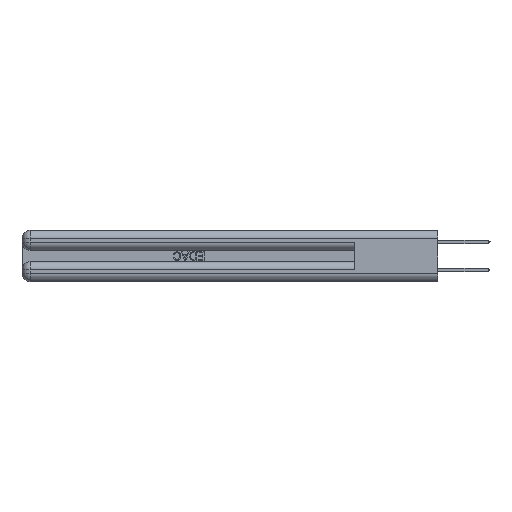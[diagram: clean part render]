
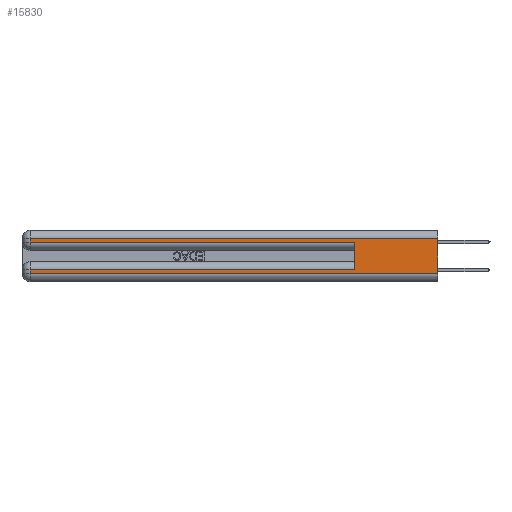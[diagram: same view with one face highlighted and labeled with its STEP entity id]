
A CAD part, left-side view. The second image highlights one B-rep face of the part: STEP entity #15830.
In plain terms, the highlighted planar face has unit normal (-1, 0, 0).
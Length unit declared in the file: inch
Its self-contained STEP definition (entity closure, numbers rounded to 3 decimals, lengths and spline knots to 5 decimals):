
#198 = DIRECTION ( 'NONE',  ( 1., 0., 0. ) ) ;
#2492 = DIRECTION ( 'NONE',  ( 0., 0., -1. ) ) ;
#3030 = CARTESIAN_POINT ( 'NONE',  ( 0., 2.94, 0.31 ) ) ;
#3040 = LINE ( 'NONE', #41547, #27461 ) ;
#3312 = EDGE_CURVE ( 'NONE', #23851, #37595, #28689, .T. ) ;
#4553 = CARTESIAN_POINT ( 'NONE',  ( 0., 0.6, 0.285 ) ) ;
#5303 = VECTOR ( 'NONE', #10422, 39.37008 ) ;
#5390 = LINE ( 'NONE', #34972, #40465 ) ;
#6276 = LINE ( 'NONE', #22838, #38708 ) ;
#8292 = LINE ( 'NONE', #35567, #41239 ) ;
#8572 = ORIENTED_EDGE ( 'NONE', *, *, #43163, .T. ) ;
#9843 = CARTESIAN_POINT ( 'NONE',  ( 0., 0., 0.06 ) ) ;
#9988 = PLANE ( 'NONE',  #39927 ) ;
#10325 = ORIENTED_EDGE ( 'NONE', *, *, #29153, .T. ) ;
#10422 = DIRECTION ( 'NONE',  ( 0., -1., 0. ) ) ;
#10714 = CARTESIAN_POINT ( 'NONE',  ( 0., 2.94, 0.06 ) ) ;
#12516 = ORIENTED_EDGE ( 'NONE', *, *, #3312, .F. ) ;
#13775 = LINE ( 'NONE', #9843, #5303 ) ;
#14631 = DIRECTION ( 'NONE',  ( 0., -1., 0. ) ) ;
#15467 = VERTEX_POINT ( 'NONE', #18039 ) ;
#15791 = VECTOR ( 'NONE', #17894, 39.37008 ) ;
#15810 = VERTEX_POINT ( 'NONE', #36721 ) ;
#15830 = ADVANCED_FACE ( 'NONE', ( #37527 ), #9988, .F. ) ;
#16355 = LINE ( 'NONE', #16717, #15791 ) ;
#16717 = CARTESIAN_POINT ( 'NONE',  ( 0., 0., 0.085 ) ) ;
#17244 = CARTESIAN_POINT ( 'NONE',  ( 0., 0., 0.37 ) ) ;
#17389 = VERTEX_POINT ( 'NONE', #3030 ) ;
#17894 = DIRECTION ( 'NONE',  ( 0., 1., 0. ) ) ;
#18039 = CARTESIAN_POINT ( 'NONE',  ( 0., 0., 0.06 ) ) ;
#18085 = VERTEX_POINT ( 'NONE', #10714 ) ;
#18090 = LINE ( 'NONE', #30575, #23398 ) ;
#18903 = DIRECTION ( 'NONE',  ( 0., 1., 0. ) ) ;
#19079 = EDGE_CURVE ( 'NONE', #17389, #15810, #18090, .T. ) ;
#19759 = EDGE_LOOP ( 'NONE', ( #37384, #10325, #24664, #42009, #12516, #8572, #40927, #27533 ) ) ;
#20615 = EDGE_CURVE ( 'NONE', #32021, #18085, #6276, .T. ) ;
#21072 = EDGE_CURVE ( 'NONE', #33374, #15467, #3040, .T. ) ;
#22838 = CARTESIAN_POINT ( 'NONE',  ( 0., 2.94, 0.37 ) ) ;
#23238 = CARTESIAN_POINT ( 'NONE',  ( 0., 0.6, 0.085 ) ) ;
#23398 = VECTOR ( 'NONE', #37446, 39.37008 ) ;
#23851 = VERTEX_POINT ( 'NONE', #23238 ) ;
#24664 = ORIENTED_EDGE ( 'NONE', *, *, #19079, .T. ) ;
#24720 = DIRECTION ( 'NONE',  ( 0., 0., 1. ) ) ;
#26975 = EDGE_CURVE ( 'NONE', #15810, #37595, #5390, .T. ) ;
#27461 = VECTOR ( 'NONE', #34554, 39.37008 ) ;
#27533 = ORIENTED_EDGE ( 'NONE', *, *, #32910, .T. ) ;
#28416 = CARTESIAN_POINT ( 'NONE',  ( 0., 0.6, 0.145 ) ) ;
#28689 = LINE ( 'NONE', #28416, #35643 ) ;
#29153 = EDGE_CURVE ( 'NONE', #33374, #17389, #8292, .T. ) ;
#29156 = CARTESIAN_POINT ( 'NONE',  ( 0., 2.94, 0.085 ) ) ;
#30575 = CARTESIAN_POINT ( 'NONE',  ( 0., 2.94, 0.37 ) ) ;
#32021 = VERTEX_POINT ( 'NONE', #29156 ) ;
#32910 = EDGE_CURVE ( 'NONE', #18085, #15467, #13775, .T. ) ;
#33374 = VERTEX_POINT ( 'NONE', #36760 ) ;
#33884 = DIRECTION ( 'NONE',  ( 0., 0., -1. ) ) ;
#34554 = DIRECTION ( 'NONE',  ( 0., 0., -1. ) ) ;
#34972 = CARTESIAN_POINT ( 'NONE',  ( 0., 0., 0.285 ) ) ;
#35567 = CARTESIAN_POINT ( 'NONE',  ( 0., 0., 0.31 ) ) ;
#35643 = VECTOR ( 'NONE', #24720, 39.37008 ) ;
#36721 = CARTESIAN_POINT ( 'NONE',  ( 0., 2.94, 0.285 ) ) ;
#36760 = CARTESIAN_POINT ( 'NONE',  ( 0., 0., 0.31 ) ) ;
#37384 = ORIENTED_EDGE ( 'NONE', *, *, #21072, .F. ) ;
#37446 = DIRECTION ( 'NONE',  ( 0., 0., -1. ) ) ;
#37527 = FACE_OUTER_BOUND ( 'NONE', #19759, .T. ) ;
#37595 = VERTEX_POINT ( 'NONE', #4553 ) ;
#38708 = VECTOR ( 'NONE', #2492, 39.37008 ) ;
#39927 = AXIS2_PLACEMENT_3D ( 'NONE', #17244, #198, #33884 ) ;
#40465 = VECTOR ( 'NONE', #14631, 39.37008 ) ;
#40927 = ORIENTED_EDGE ( 'NONE', *, *, #20615, .T. ) ;
#41239 = VECTOR ( 'NONE', #18903, 39.37008 ) ;
#41547 = CARTESIAN_POINT ( 'NONE',  ( 0., 0., 0.37 ) ) ;
#42009 = ORIENTED_EDGE ( 'NONE', *, *, #26975, .T. ) ;
#43163 = EDGE_CURVE ( 'NONE', #23851, #32021, #16355, .T. ) ;
